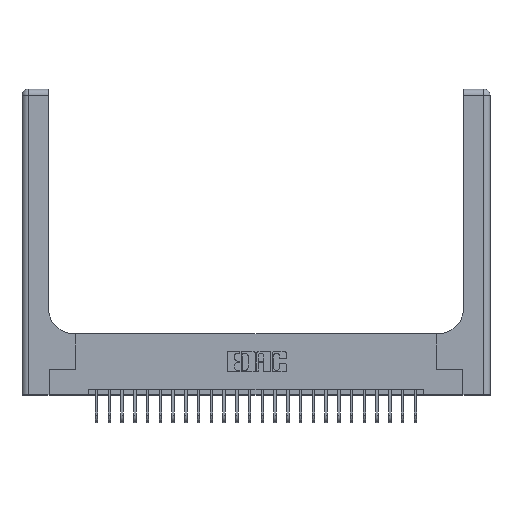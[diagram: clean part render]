
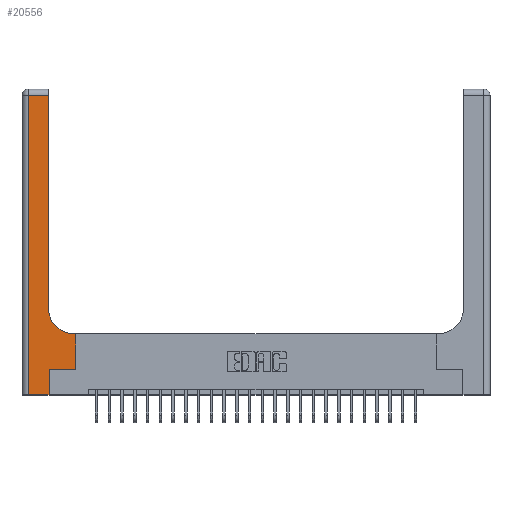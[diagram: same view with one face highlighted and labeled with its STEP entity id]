
A CAD part, top view. The second image highlights one B-rep face of the part: STEP entity #20556.
In plain terms, the highlighted planar face has unit normal (0, 0, 1).
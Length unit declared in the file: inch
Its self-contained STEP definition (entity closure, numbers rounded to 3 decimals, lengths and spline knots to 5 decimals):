
#421 = EDGE_CURVE ( 'NONE', #19916, #14697, #4303, .T. ) ;
#545 = DIRECTION ( 'NONE',  ( 1., 0., 0. ) ) ;
#803 = ORIENTED_EDGE ( 'NONE', *, *, #5412, .T. ) ;
#870 = VERTEX_POINT ( 'NONE', #2360 ) ;
#951 = VECTOR ( 'NONE', #20730, 39.37008 ) ;
#1247 = CARTESIAN_POINT ( 'NONE',  ( 0.26, 0.6, 0.37 ) ) ;
#1294 = AXIS2_PLACEMENT_3D ( 'NONE', #6307, #16924, #4550 ) ;
#1301 = DIRECTION ( 'NONE',  ( 1., 0., 0. ) ) ;
#1380 = ORIENTED_EDGE ( 'NONE', *, *, #8156, .T. ) ;
#2275 = PLANE ( 'NONE',  #1294 ) ;
#2294 = CARTESIAN_POINT ( 'NONE',  ( 0.26, 3., 0.37 ) ) ;
#2296 = DIRECTION ( 'NONE',  ( -1., 0., 0. ) ) ;
#2300 = VECTOR ( 'NONE', #1301, 39.37008 ) ;
#2360 = CARTESIAN_POINT ( 'NONE',  ( 0.06, 0., 0.37 ) ) ;
#2544 = LINE ( 'NONE', #4304, #9457 ) ;
#2554 = LINE ( 'NONE', #6735, #3241 ) ;
#2877 = EDGE_CURVE ( 'NONE', #4975, #22920, #2554, .T. ) ;
#3241 = VECTOR ( 'NONE', #545, 39.37008 ) ;
#3663 = EDGE_CURVE ( 'NONE', #870, #15861, #21986, .T. ) ;
#3810 = DIRECTION ( 'NONE',  ( 0., 1., 0. ) ) ;
#3921 = CIRCLE ( 'NONE', #7343, 0.25 ) ;
#4038 = DIRECTION ( 'NONE',  ( 0., 1., 0. ) ) ;
#4303 = LINE ( 'NONE', #2294, #15017 ) ;
#4304 = CARTESIAN_POINT ( 'NONE',  ( 0., 2.94, 0.37 ) ) ;
#4550 = DIRECTION ( 'NONE',  ( -1., 0., 0. ) ) ;
#4975 = VERTEX_POINT ( 'NONE', #7907 ) ;
#5412 = EDGE_CURVE ( 'NONE', #22920, #23585, #7983, .T. ) ;
#5826 = CARTESIAN_POINT ( 'NONE',  ( 0.528, 0.25, 0.37 ) ) ;
#5848 = EDGE_CURVE ( 'NONE', #14697, #19302, #2544, .T. ) ;
#5932 = CARTESIAN_POINT ( 'NONE',  ( 0.265, 0., 0.37 ) ) ;
#6082 = LINE ( 'NONE', #16584, #951 ) ;
#6307 = CARTESIAN_POINT ( 'NONE',  ( 0., 3., 0.37 ) ) ;
#6549 = EDGE_CURVE ( 'NONE', #24662, #19916, #3921, .T. ) ;
#6567 = ORIENTED_EDGE ( 'NONE', *, *, #21164, .T. ) ;
#6735 = CARTESIAN_POINT ( 'NONE',  ( 0.265, 0.25, 0.37 ) ) ;
#7343 = AXIS2_PLACEMENT_3D ( 'NONE', #22909, #18763, #10424 ) ;
#7668 = CARTESIAN_POINT ( 'NONE',  ( 0.528, 0.25, 0.37 ) ) ;
#7907 = CARTESIAN_POINT ( 'NONE',  ( 0.265, 0.25, 0.37 ) ) ;
#7983 = LINE ( 'NONE', #5826, #10731 ) ;
#8156 = EDGE_CURVE ( 'NONE', #19302, #870, #6082, .T. ) ;
#8726 = LINE ( 'NONE', #16947, #23695 ) ;
#9324 = EDGE_LOOP ( 'NONE', ( #9474, #21983, #1380, #22202, #15558, #12829, #803, #6567, #20906 ) ) ;
#9415 = CARTESIAN_POINT ( 'NONE',  ( 0.51, 0.6, 0.37 ) ) ;
#9457 = VECTOR ( 'NONE', #2296, 39.37008 ) ;
#9474 = ORIENTED_EDGE ( 'NONE', *, *, #421, .T. ) ;
#9567 = DIRECTION ( 'NONE',  ( -1., 0., 0. ) ) ;
#9884 = EDGE_CURVE ( 'NONE', #15861, #4975, #8726, .T. ) ;
#10424 = DIRECTION ( 'NONE',  ( 1., 0., 0. ) ) ;
#10731 = VECTOR ( 'NONE', #3810, 39.37008 ) ;
#12829 = ORIENTED_EDGE ( 'NONE', *, *, #2877, .T. ) ;
#13017 = CARTESIAN_POINT ( 'NONE',  ( 0.26, 2.94, 0.37 ) ) ;
#14697 = VERTEX_POINT ( 'NONE', #13017 ) ;
#15017 = VECTOR ( 'NONE', #4038, 39.37008 ) ;
#15054 = VECTOR ( 'NONE', #9567, 39.37008 ) ;
#15558 = ORIENTED_EDGE ( 'NONE', *, *, #9884, .T. ) ;
#15861 = VERTEX_POINT ( 'NONE', #5932 ) ;
#16584 = CARTESIAN_POINT ( 'NONE',  ( 0.06, 3., 0.37 ) ) ;
#16924 = DIRECTION ( 'NONE',  ( 0., 0., -1. ) ) ;
#16947 = CARTESIAN_POINT ( 'NONE',  ( 0.265, 0., 0.37 ) ) ;
#18763 = DIRECTION ( 'NONE',  ( 0., 0., -1. ) ) ;
#18922 = FACE_OUTER_BOUND ( 'NONE', #9324, .T. ) ;
#19302 = VERTEX_POINT ( 'NONE', #21024 ) ;
#19916 = VERTEX_POINT ( 'NONE', #23628 ) ;
#20556 = ADVANCED_FACE ( 'NONE', ( #18922 ), #2275, .F. ) ;
#20730 = DIRECTION ( 'NONE',  ( 0., -1., 0. ) ) ;
#20786 = CARTESIAN_POINT ( 'NONE',  ( 0.528, 0.6, 0.37 ) ) ;
#20906 = ORIENTED_EDGE ( 'NONE', *, *, #6549, .T. ) ;
#21024 = CARTESIAN_POINT ( 'NONE',  ( 0.06, 2.94, 0.37 ) ) ;
#21164 = EDGE_CURVE ( 'NONE', #23585, #24662, #22070, .T. ) ;
#21723 = CARTESIAN_POINT ( 'NONE',  ( 0., 0., 0.37 ) ) ;
#21983 = ORIENTED_EDGE ( 'NONE', *, *, #5848, .T. ) ;
#21986 = LINE ( 'NONE', #21723, #2300 ) ;
#22070 = LINE ( 'NONE', #1247, #15054 ) ;
#22202 = ORIENTED_EDGE ( 'NONE', *, *, #3663, .T. ) ;
#22909 = CARTESIAN_POINT ( 'NONE',  ( 0.51, 0.85, 0.37 ) ) ;
#22920 = VERTEX_POINT ( 'NONE', #7668 ) ;
#23585 = VERTEX_POINT ( 'NONE', #20786 ) ;
#23628 = CARTESIAN_POINT ( 'NONE',  ( 0.26, 0.85, 0.37 ) ) ;
#23695 = VECTOR ( 'NONE', #25125, 39.37008 ) ;
#24662 = VERTEX_POINT ( 'NONE', #9415 ) ;
#25125 = DIRECTION ( 'NONE',  ( 0., 1., 0. ) ) ;
